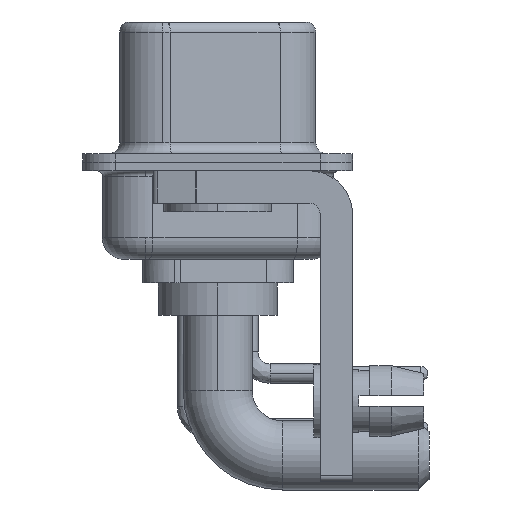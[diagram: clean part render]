
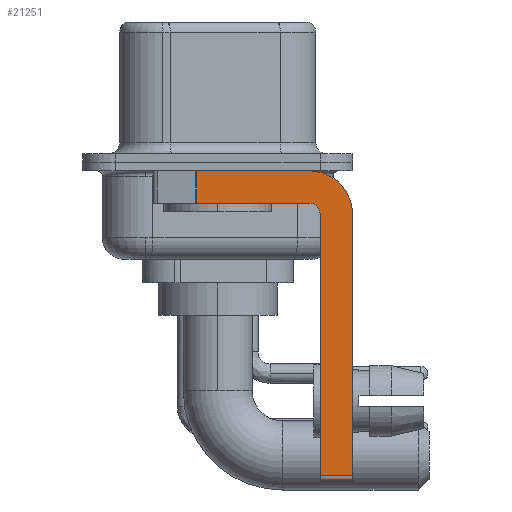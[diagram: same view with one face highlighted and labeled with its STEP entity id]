
A CAD part, left-side view. The second image highlights one B-rep face of the part: STEP entity #21251.
In plain terms, the highlighted planar face has unit normal (-1, 0, 0).
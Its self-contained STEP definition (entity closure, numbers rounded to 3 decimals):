
#324 = AXIS2_PLACEMENT_3D ( 'NONE', #2501, #2766, #10910 ) ;
#641 = CARTESIAN_POINT ( 'NONE',  ( -2.9, -6.25, -14.55 ) ) ;
#669 = DIRECTION ( 'NONE',  ( 1., 0., 0. ) ) ;
#2419 = DIRECTION ( 'NONE',  ( 0., 1., 0. ) ) ;
#2501 = CARTESIAN_POINT ( 'NONE',  ( -2.9, -4.25, -2.4 ) ) ;
#2766 = DIRECTION ( 'NONE',  ( -1., 0., 0. ) ) ;
#4011 = CARTESIAN_POINT ( 'NONE',  ( -2.9, -6.25, -2.4 ) ) ;
#5170 = ORIENTED_EDGE ( 'NONE', *, *, #14397, .F. ) ;
#5344 = EDGE_CURVE ( 'NONE', #25229, #20954, #9426, .T. ) ;
#5390 = ORIENTED_EDGE ( 'NONE', *, *, #8326, .F. ) ;
#6000 = CARTESIAN_POINT ( 'NONE',  ( -2.9, -4.25, -0.4 ) ) ;
#7175 = EDGE_CURVE ( 'NONE', #17038, #18687, #10701, .T. ) ;
#7237 = AXIS2_PLACEMENT_3D ( 'NONE', #19169, #669, #23397 ) ;
#8326 = EDGE_CURVE ( 'NONE', #25229, #16755, #9544, .T. ) ;
#9423 = EDGE_CURVE ( 'NONE', #24541, #15151, #23789, .T. ) ;
#9426 = LINE ( 'NONE', #15960, #13451 ) ;
#9544 = LINE ( 'NONE', #25878, #12509 ) ;
#9591 = VERTEX_POINT ( 'NONE', #17862 ) ;
#9969 = CARTESIAN_POINT ( 'NONE',  ( -2.9, 0.978, -0.4 ) ) ;
#10701 = LINE ( 'NONE', #12346, #13543 ) ;
#10862 = LINE ( 'NONE', #23532, #23164 ) ;
#10910 = DIRECTION ( 'NONE',  ( 0., 0., 1. ) ) ;
#11048 = EDGE_CURVE ( 'NONE', #17038, #24541, #10862, .T. ) ;
#11978 = EDGE_LOOP ( 'NONE', ( #5390, #25736, #20441, #22560, #16700, #25410, #12120, #5170 ) ) ;
#12120 = ORIENTED_EDGE ( 'NONE', *, *, #13160, .F. ) ;
#12346 = CARTESIAN_POINT ( 'NONE',  ( -2.9, -4.25, -14.55 ) ) ;
#12509 = VECTOR ( 'NONE', #13766, 1000. ) ;
#12877 = LINE ( 'NONE', #15066, #23845 ) ;
#13160 = EDGE_CURVE ( 'NONE', #9591, #18687, #18591, .T. ) ;
#13451 = VECTOR ( 'NONE', #24264, 1000. ) ;
#13521 = CARTESIAN_POINT ( 'NONE',  ( -2.9, -4.25, -2.4 ) ) ;
#13543 = VECTOR ( 'NONE', #24606, 1000. ) ;
#13766 = DIRECTION ( 'NONE',  ( 0., -1., 0. ) ) ;
#14397 = EDGE_CURVE ( 'NONE', #16755, #9591, #19417, .T. ) ;
#14857 = AXIS2_PLACEMENT_3D ( 'NONE', #13521, #15979, #21565 ) ;
#15066 = CARTESIAN_POINT ( 'NONE',  ( -2.9, -4.25, -1.9 ) ) ;
#15151 = VERTEX_POINT ( 'NONE', #15260 ) ;
#15260 = CARTESIAN_POINT ( 'NONE',  ( -2.9, -4.25, -1.9 ) ) ;
#15480 = CARTESIAN_POINT ( 'NONE',  ( -2.9, -4.75, -2.4 ) ) ;
#15580 = PLANE ( 'NONE',  #14857 ) ;
#15960 = CARTESIAN_POINT ( 'NONE',  ( -2.9, 0.978, -1.9 ) ) ;
#15979 = DIRECTION ( 'NONE',  ( 1., 0., 0. ) ) ;
#16700 = ORIENTED_EDGE ( 'NONE', *, *, #11048, .F. ) ;
#16755 = VERTEX_POINT ( 'NONE', #6000 ) ;
#17038 = VERTEX_POINT ( 'NONE', #25603 ) ;
#17392 = EDGE_CURVE ( 'NONE', #15151, #20954, #12877, .T. ) ;
#17862 = CARTESIAN_POINT ( 'NONE',  ( -2.9, -6.25, -2.4 ) ) ;
#18591 = LINE ( 'NONE', #4011, #21530 ) ;
#18687 = VERTEX_POINT ( 'NONE', #641 ) ;
#19169 = CARTESIAN_POINT ( 'NONE',  ( -2.9, -4.25, -2.4 ) ) ;
#19417 = CIRCLE ( 'NONE', #7237, 2. ) ;
#19782 = FACE_OUTER_BOUND ( 'NONE', #11978, .T. ) ;
#20441 = ORIENTED_EDGE ( 'NONE', *, *, #17392, .F. ) ;
#20954 = VERTEX_POINT ( 'NONE', #24835 ) ;
#21251 = ADVANCED_FACE ( 'NONE', ( #19782 ), #15580, .F. ) ;
#21530 = VECTOR ( 'NONE', #22941, 1000. ) ;
#21565 = DIRECTION ( 'NONE',  ( 0., 0., -1. ) ) ;
#21629 = DIRECTION ( 'NONE',  ( 0., 0., 1. ) ) ;
#22560 = ORIENTED_EDGE ( 'NONE', *, *, #9423, .F. ) ;
#22941 = DIRECTION ( 'NONE',  ( 0., 0., -1. ) ) ;
#23164 = VECTOR ( 'NONE', #21629, 1000. ) ;
#23397 = DIRECTION ( 'NONE',  ( 0., 0., -1. ) ) ;
#23532 = CARTESIAN_POINT ( 'NONE',  ( -2.9, -4.75, -14.8 ) ) ;
#23789 = CIRCLE ( 'NONE', #324, 0.5 ) ;
#23845 = VECTOR ( 'NONE', #2419, 1000. ) ;
#24264 = DIRECTION ( 'NONE',  ( 0., 0., -1. ) ) ;
#24541 = VERTEX_POINT ( 'NONE', #15480 ) ;
#24606 = DIRECTION ( 'NONE',  ( 0., -1., 0. ) ) ;
#24835 = CARTESIAN_POINT ( 'NONE',  ( -2.9, 0.978, -1.9 ) ) ;
#25229 = VERTEX_POINT ( 'NONE', #9969 ) ;
#25410 = ORIENTED_EDGE ( 'NONE', *, *, #7175, .T. ) ;
#25603 = CARTESIAN_POINT ( 'NONE',  ( -2.9, -4.75, -14.55 ) ) ;
#25736 = ORIENTED_EDGE ( 'NONE', *, *, #5344, .T. ) ;
#25878 = CARTESIAN_POINT ( 'NONE',  ( -2.9, 3., -0.4 ) ) ;
